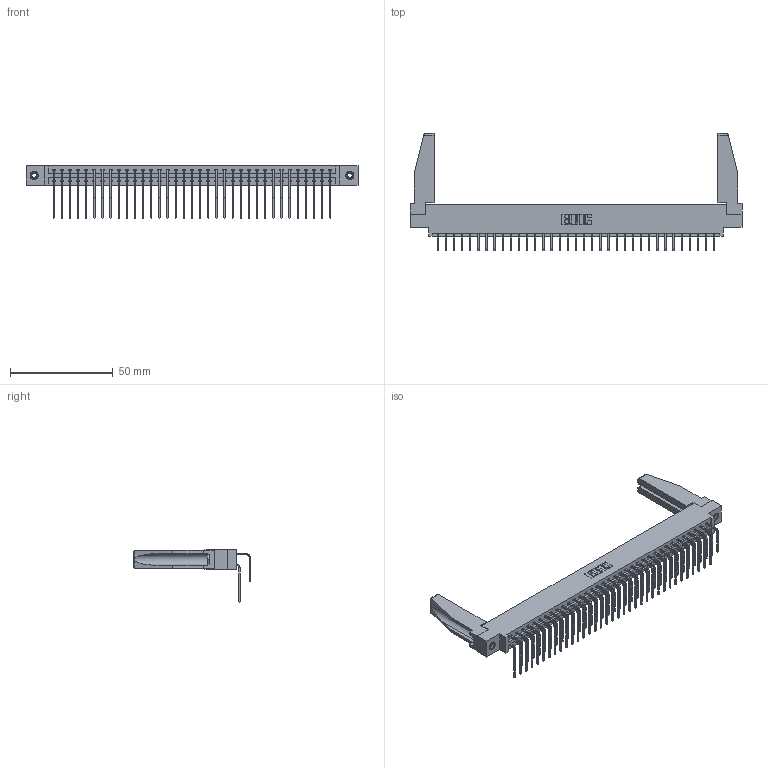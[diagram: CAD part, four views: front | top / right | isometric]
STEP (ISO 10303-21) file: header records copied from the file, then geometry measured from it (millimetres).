
FILE_DESCRIPTION (( 'STEP AP203' ), '1' );
FILE_NAME ('387-070-558-878.STEP', '2019-10-21T23:08:24', ( '' ), ( '' ), 'SwSTEP 2.0', 'SolidWorks 2016', '' );
FILE_SCHEMA (( 'CONFIG_CONTROL_DESIGN' ));
Length unit declared in the file: inch
Products named in the file (6): 307-220-078; 337 Part_0.170 Offset - 0.156 Dia-TI; 387-070-558-878; 345-292-001_558 Tail - 2; 345-250-001_345-250-001-102; 345-292-001_558 559 Tail - 1
Assembly tree (75 placements, depth 2):
  387-070-558-878
    337 Part_0.170 Offset - 0.156 Dia-TI
    345-292-001_558 559 Tail - 1  x35
    345-292-001_558 Tail - 2  x35
    345-250-001_345-250-001-102  x2
    307-220-078  x2
Bounding box: 161.7 x 56.96 x 25.53 mm (x, y, z)
Volume: 21227.3 mm3; surface area: 25381 mm2
Topology: 75 solids, 75 shells, 4168 faces, 12343 edges, 8126 vertices
Faces by surface type: plane 2958, cylinder 1194, cone 12, torus 4
Entity records: 32398 total; most frequent: CARTESIAN_POINT 5511, ORIENTED_EDGE 5352, DIRECTION 4688, EDGE_CURVE 2676, VECTOR 2470, LINE 2470, VERTEX_POINT 1776, AXIS2_PLACEMENT_3D 1109
